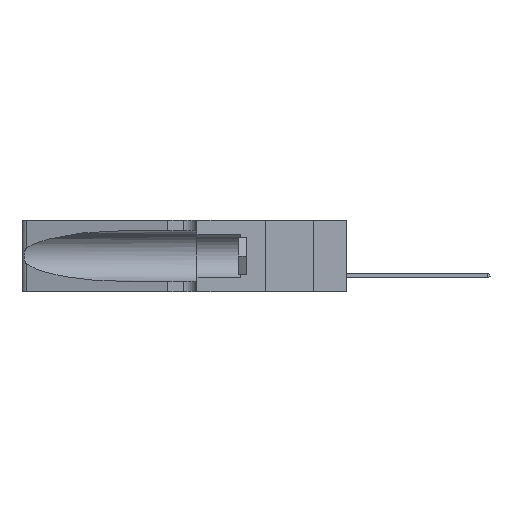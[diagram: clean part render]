
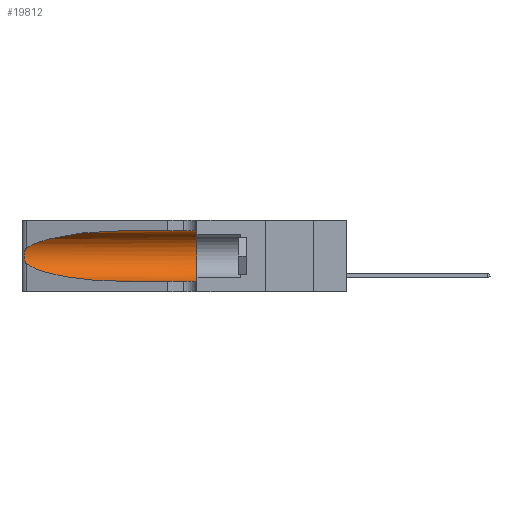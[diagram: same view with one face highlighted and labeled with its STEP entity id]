
A CAD part, left-side view. The second image highlights one B-rep face of the part: STEP entity #19812.
In plain terms, the highlighted cylindrical face has radius 3.308 mm (diameter 6.617 mm), a partial arc.
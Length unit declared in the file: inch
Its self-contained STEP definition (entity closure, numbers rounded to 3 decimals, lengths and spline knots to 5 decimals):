
#860 = EDGE_CURVE ( 'NONE', #20991, #22212, #15102, .T. ) ;
#921 = CARTESIAN_POINT ( 'NONE',  ( 0.25487, 1.22718, 0.22369 ) ) ;
#1056 = CARTESIAN_POINT ( 'NONE',  ( 0.25854, 1.2359, 0.20912 ) ) ;
#1231 = CARTESIAN_POINT ( 'NONE',  ( 0.25639, 1.23184, 0.21858 ) ) ;
#2905 = CARTESIAN_POINT ( 'NONE',  ( 0.26075, 1.23896, 0.178 ) ) ;
#3245 = CARTESIAN_POINT ( 'NONE',  ( 0.26075, 1.23896, 0.19203 ) ) ;
#3464 = ORIENTED_EDGE ( 'NONE', *, *, #10687, .F. ) ;
#3572 = CARTESIAN_POINT ( 'NONE',  ( 0.25639, 1.23186, 0.15144 ) ) ;
#3651 = CARTESIAN_POINT ( 'NONE',  ( 0.25487, 1.22718, 0.14631 ) ) ;
#4286 = CARTESIAN_POINT ( 'NONE',  ( 0.1305, 1.61858, 0.05475 ) ) ;
#4287 = ORIENTED_EDGE ( 'NONE', *, *, #860, .T. ) ;
#4299 = CARTESIAN_POINT ( 'NONE',  ( 0.25487, 1.22718, 0.14631 ) ) ;
#4812 = CARTESIAN_POINT ( 'NONE',  ( 0.26017, 1.23833, 0.17102 ) ) ;
#5746 = ORIENTED_EDGE ( 'NONE', *, *, #9877, .F. ) ;
#6059 = VERTEX_POINT ( 'NONE', #15005 ) ;
#6784 = DIRECTION ( 'NONE',  ( 0., 0., -1. ) ) ;
#6935 = CARTESIAN_POINT ( 'NONE',  ( 0.25487, 1.22718, 0.22369 ) ) ;
#7034 = CARTESIAN_POINT ( 'NONE',  ( 0.25856, 1.23593, 0.16098 ) ) ;
#7063 = CARTESIAN_POINT ( 'NONE',  ( 0.1305, 0.72297, 0.31525 ) ) ;
#7178 = DIRECTION ( 'NONE',  ( 0., -1., 0. ) ) ;
#7639 = VERTEX_POINT ( 'NONE', #12053 ) ;
#8288 = EDGE_CURVE ( 'NONE', #16991, #7639, #19732, .T. ) ;
#8434 = B_SPLINE_CURVE_WITH_KNOTS ( 'NONE', 3,
 ( #6935, #12817, #1231, #12555, #1056, #14745, #3245, #2905, #4812, #7034, #20785, #3572, #17099, #3651 ),
 .UNSPECIFIED., .F., .F.,
 ( 4, 2, 2, 2, 2, 2, 4 ),
 ( 0., 0.00027, 0.00053, 0.00107, 0.0016, 0.00187, 0.00214 ),
 .UNSPECIFIED. ) ;
#8893 = LINE ( 'NONE', #12788, #10076 ) ;
#8921 = CYLINDRICAL_SURFACE ( 'NONE', #16943, 0.13025 ) ;
#9389 = DIRECTION ( 'NONE',  ( 0., 0., 1. ) ) ;
#9482 = ORIENTED_EDGE ( 'NONE', *, *, #21630, .T. ) ;
#9877 = EDGE_CURVE ( 'NONE', #20991, #6059, #8893, .T. ) ;
#10076 = VECTOR ( 'NONE', #7178, 39.37008 ) ;
#10687 = EDGE_CURVE ( 'NONE', #6059, #10838, #13932, .T. ) ;
#10838 = VERTEX_POINT ( 'NONE', #22824 ) ;
#11216 = CARTESIAN_POINT ( 'NONE',  ( 0.1305, 0.35, 0.185 ) ) ;
#11457 = ORIENTED_EDGE ( 'NONE', *, *, #14517, .T. ) ;
#12053 = CARTESIAN_POINT ( 'NONE',  ( 0.1305, 0.72297, 0.05475 ) ) ;
#12555 = CARTESIAN_POINT ( 'NONE',  ( 0.25787, 1.23484, 0.2124 ) ) ;
#12788 = CARTESIAN_POINT ( 'NONE',  ( 0.1305, 1.61858, 0.31525 ) ) ;
#12817 = CARTESIAN_POINT ( 'NONE',  ( 0.25555, 1.22994, 0.2215 ) ) ;
#13886 = CARTESIAN_POINT ( 'NONE',  ( 0.2373, 1.15595, 0.08982 ) ) ;
#13932 = CIRCLE ( 'NONE', #21836, 0.13025 ) ;
#14508 = DIRECTION ( 'NONE',  ( 0., -1., 0. ) ) ;
#14517 = EDGE_CURVE ( 'NONE', #7639, #10838, #23019, .T. ) ;
#14745 = CARTESIAN_POINT ( 'NONE',  ( 0.26018, 1.23835, 0.19895 ) ) ;
#15005 = CARTESIAN_POINT ( 'NONE',  ( 0.1305, 0.35, 0.31525 ) ) ;
#15102 =( BOUNDED_CURVE ( )  B_SPLINE_CURVE ( 3, ( #17768, #24961, #22082, #921 ),
 .UNSPECIFIED., .F., .F. ) 
 B_SPLINE_CURVE_WITH_KNOTS ( ( 4, 4 ),
 ( 1.5708, 2.84003 ),
 .UNSPECIFIED. ) 
 CURVE ( )  GEOMETRIC_REPRESENTATION_ITEM ( )  RATIONAL_B_SPLINE_CURVE ( ( 1., 0.87, 0.87, 1. ) ) 
 REPRESENTATION_ITEM ( '' )  );
#16144 = ORIENTED_EDGE ( 'NONE', *, *, #8288, .T. ) ;
#16943 = AXIS2_PLACEMENT_3D ( 'NONE', #20282, #14508, #6784 ) ;
#16991 = VERTEX_POINT ( 'NONE', #18008 ) ;
#17099 = CARTESIAN_POINT ( 'NONE',  ( 0.25555, 1.22993, 0.14849 ) ) ;
#17671 = DIRECTION ( 'NONE',  ( 0., -1., 0. ) ) ;
#17680 = CARTESIAN_POINT ( 'NONE',  ( 0.1305, 0.72297, 0.05475 ) ) ;
#17768 = CARTESIAN_POINT ( 'NONE',  ( 0.1305, 0.72297, 0.31525 ) ) ;
#17831 = VECTOR ( 'NONE', #17671, 39.37008 ) ;
#18008 = CARTESIAN_POINT ( 'NONE',  ( 0.25487, 1.22718, 0.14631 ) ) ;
#18092 = CARTESIAN_POINT ( 'NONE',  ( 0.25487, 1.22718, 0.22369 ) ) ;
#19732 =( BOUNDED_CURVE ( )  B_SPLINE_CURVE ( 3, ( #4299, #13886, #19816, #17680 ),
 .UNSPECIFIED., .F., .T. ) 
 B_SPLINE_CURVE_WITH_KNOTS ( ( 4, 4 ),
 ( 3.44316, 4.71239 ),
 .UNSPECIFIED. ) 
 CURVE ( )  GEOMETRIC_REPRESENTATION_ITEM ( )  RATIONAL_B_SPLINE_CURVE ( ( 1., 0.87, 0.87, 1. ) ) 
 REPRESENTATION_ITEM ( '' )  );
#19812 = ADVANCED_FACE ( 'NONE', ( #23452 ), #8921, .F. ) ;
#19816 = CARTESIAN_POINT ( 'NONE',  ( 0.18966, 0.96281, 0.05475 ) ) ;
#20282 = CARTESIAN_POINT ( 'NONE',  ( 0.1305, 1.61858, 0.185 ) ) ;
#20785 = CARTESIAN_POINT ( 'NONE',  ( 0.25789, 1.23486, 0.15765 ) ) ;
#20961 = DIRECTION ( 'NONE',  ( 0., 1., 0. ) ) ;
#20991 = VERTEX_POINT ( 'NONE', #7063 ) ;
#21630 = EDGE_CURVE ( 'NONE', #22212, #16991, #8434, .T. ) ;
#21836 = AXIS2_PLACEMENT_3D ( 'NONE', #11216, #20961, #9389 ) ;
#22082 = CARTESIAN_POINT ( 'NONE',  ( 0.2373, 1.15595, 0.28018 ) ) ;
#22212 = VERTEX_POINT ( 'NONE', #18092 ) ;
#22824 = CARTESIAN_POINT ( 'NONE',  ( 0.1305, 0.35, 0.05475 ) ) ;
#23019 = LINE ( 'NONE', #4286, #17831 ) ;
#23452 = FACE_OUTER_BOUND ( 'NONE', #23562, .T. ) ;
#23562 = EDGE_LOOP ( 'NONE', ( #4287, #9482, #16144, #11457, #3464, #5746 ) ) ;
#24961 = CARTESIAN_POINT ( 'NONE',  ( 0.18966, 0.96281, 0.31525 ) ) ;
